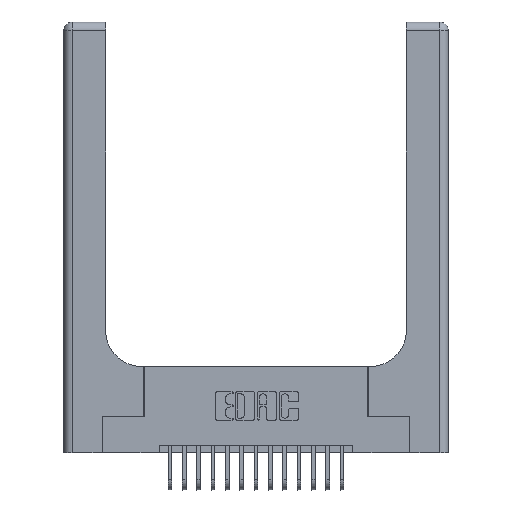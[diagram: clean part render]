
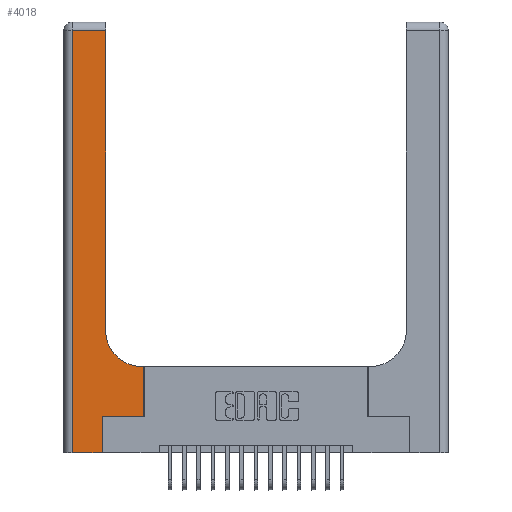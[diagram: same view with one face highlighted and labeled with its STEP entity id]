
A CAD part, top view. The second image highlights one B-rep face of the part: STEP entity #4018.
In plain terms, the highlighted planar face has unit normal (0, 0, 1).
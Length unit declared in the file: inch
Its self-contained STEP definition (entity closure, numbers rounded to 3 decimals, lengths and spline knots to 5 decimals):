
#13 = EDGE_LOOP ( 'NONE', ( #11872, #17772, #3236, #15732, #1699, #1642, #19374, #10891, #4149 ) ) ;
#939 = LINE ( 'NONE', #1383, #10527 ) ;
#1269 = CARTESIAN_POINT ( 'NONE',  ( 0.269, 0., 0.37 ) ) ;
#1286 = VERTEX_POINT ( 'NONE', #3734 ) ;
#1312 = CARTESIAN_POINT ( 'NONE',  ( 0.269, 0., 0.37 ) ) ;
#1383 = CARTESIAN_POINT ( 'NONE',  ( 0.06, 3., 0.37 ) ) ;
#1642 = ORIENTED_EDGE ( 'NONE', *, *, #1712, .T. ) ;
#1699 = ORIENTED_EDGE ( 'NONE', *, *, #9197, .T. ) ;
#1712 = EDGE_CURVE ( 'NONE', #12130, #8236, #8034, .T. ) ;
#1850 = EDGE_CURVE ( 'NONE', #14033, #8710, #14311, .T. ) ;
#2122 = LINE ( 'NONE', #20384, #19848 ) ;
#2310 = LINE ( 'NONE', #8805, #19551 ) ;
#2671 = VECTOR ( 'NONE', #16369, 39.37008 ) ;
#2741 = DIRECTION ( 'NONE',  ( 0., 1., 0. ) ) ;
#3094 = VERTEX_POINT ( 'NONE', #9055 ) ;
#3236 = ORIENTED_EDGE ( 'NONE', *, *, #11175, .T. ) ;
#3260 = LINE ( 'NONE', #1269, #10853 ) ;
#3734 = CARTESIAN_POINT ( 'NONE',  ( 0.2915, 2.94, 0.37 ) ) ;
#3889 = DIRECTION ( 'NONE',  ( 0., 1., 0. ) ) ;
#4018 = ADVANCED_FACE ( 'NONE', ( #7455 ), #13034, .F. ) ;
#4032 = CARTESIAN_POINT ( 'NONE',  ( 0.5585, 0.25, 0.37 ) ) ;
#4149 = ORIENTED_EDGE ( 'NONE', *, *, #12317, .T. ) ;
#4182 = VECTOR ( 'NONE', #13411, 39.37008 ) ;
#4594 = DIRECTION ( 'NONE',  ( -1., 0., 0. ) ) ;
#5177 = LINE ( 'NONE', #12404, #8755 ) ;
#5592 = DIRECTION ( 'NONE',  ( 1., 0., 0. ) ) ;
#6106 = DIRECTION ( 'NONE',  ( 0., -1., 0. ) ) ;
#6283 = CARTESIAN_POINT ( 'NONE',  ( 0.5585, 0.25, 0.37 ) ) ;
#6542 = DIRECTION ( 'NONE',  ( 0., 0., -1. ) ) ;
#6934 = CARTESIAN_POINT ( 'NONE',  ( 0.269, 0.25, 0.37 ) ) ;
#7040 = VERTEX_POINT ( 'NONE', #15640 ) ;
#7372 = AXIS2_PLACEMENT_3D ( 'NONE', #8258, #6542, #14500 ) ;
#7455 = FACE_OUTER_BOUND ( 'NONE', #13, .T. ) ;
#8034 = LINE ( 'NONE', #6934, #2671 ) ;
#8236 = VERTEX_POINT ( 'NONE', #4032 ) ;
#8258 = CARTESIAN_POINT ( 'NONE',  ( 0., 3., 0.37 ) ) ;
#8710 = VERTEX_POINT ( 'NONE', #13926 ) ;
#8755 = VECTOR ( 'NONE', #4594, 39.37008 ) ;
#8805 = CARTESIAN_POINT ( 'NONE',  ( 0., 0., 0.37 ) ) ;
#9055 = CARTESIAN_POINT ( 'NONE',  ( 0.2915, 0.85, 0.37 ) ) ;
#9197 = EDGE_CURVE ( 'NONE', #11696, #12130, #3260, .T. ) ;
#9245 = CARTESIAN_POINT ( 'NONE',  ( 0.269, 0.25, 0.37 ) ) ;
#9542 = VERTEX_POINT ( 'NONE', #17588 ) ;
#10390 = DIRECTION ( 'NONE',  ( 0., 0., -1. ) ) ;
#10527 = VECTOR ( 'NONE', #6106, 39.37008 ) ;
#10853 = VECTOR ( 'NONE', #17300, 39.37008 ) ;
#10891 = ORIENTED_EDGE ( 'NONE', *, *, #1850, .T. ) ;
#11175 = EDGE_CURVE ( 'NONE', #7040, #9542, #939, .T. ) ;
#11486 = LINE ( 'NONE', #6283, #18861 ) ;
#11696 = VERTEX_POINT ( 'NONE', #1312 ) ;
#11757 = CIRCLE ( 'NONE', #15813, 0.25 ) ;
#11872 = ORIENTED_EDGE ( 'NONE', *, *, #15867, .T. ) ;
#12130 = VERTEX_POINT ( 'NONE', #9245 ) ;
#12213 = EDGE_CURVE ( 'NONE', #8236, #14033, #11486, .T. ) ;
#12259 = DIRECTION ( 'NONE',  ( 1., 0., 0. ) ) ;
#12317 = EDGE_CURVE ( 'NONE', #8710, #3094, #11757, .T. ) ;
#12404 = CARTESIAN_POINT ( 'NONE',  ( 0., 2.94, 0.37 ) ) ;
#13034 = PLANE ( 'NONE',  #7372 ) ;
#13411 = DIRECTION ( 'NONE',  ( -1., 0., 0. ) ) ;
#13926 = CARTESIAN_POINT ( 'NONE',  ( 0.5415, 0.6, 0.37 ) ) ;
#14033 = VERTEX_POINT ( 'NONE', #14405 ) ;
#14311 = LINE ( 'NONE', #15301, #4182 ) ;
#14405 = CARTESIAN_POINT ( 'NONE',  ( 0.5585, 0.6, 0.37 ) ) ;
#14500 = DIRECTION ( 'NONE',  ( -1., 0., 0. ) ) ;
#15180 = EDGE_CURVE ( 'NONE', #1286, #7040, #5177, .T. ) ;
#15251 = CARTESIAN_POINT ( 'NONE',  ( 0.5415, 0.85, 0.37 ) ) ;
#15301 = CARTESIAN_POINT ( 'NONE',  ( 0.2915, 0.6, 0.37 ) ) ;
#15640 = CARTESIAN_POINT ( 'NONE',  ( 0.06, 2.94, 0.37 ) ) ;
#15732 = ORIENTED_EDGE ( 'NONE', *, *, #17044, .T. ) ;
#15813 = AXIS2_PLACEMENT_3D ( 'NONE', #15251, #10390, #5592 ) ;
#15867 = EDGE_CURVE ( 'NONE', #3094, #1286, #2122, .T. ) ;
#16369 = DIRECTION ( 'NONE',  ( 1., 0., 0. ) ) ;
#17044 = EDGE_CURVE ( 'NONE', #9542, #11696, #2310, .T. ) ;
#17300 = DIRECTION ( 'NONE',  ( 0., 1., 0. ) ) ;
#17588 = CARTESIAN_POINT ( 'NONE',  ( 0.06, 0., 0.37 ) ) ;
#17772 = ORIENTED_EDGE ( 'NONE', *, *, #15180, .T. ) ;
#18861 = VECTOR ( 'NONE', #3889, 39.37008 ) ;
#19374 = ORIENTED_EDGE ( 'NONE', *, *, #12213, .T. ) ;
#19551 = VECTOR ( 'NONE', #12259, 39.37008 ) ;
#19848 = VECTOR ( 'NONE', #2741, 39.37008 ) ;
#20384 = CARTESIAN_POINT ( 'NONE',  ( 0.2915, 3., 0.37 ) ) ;
